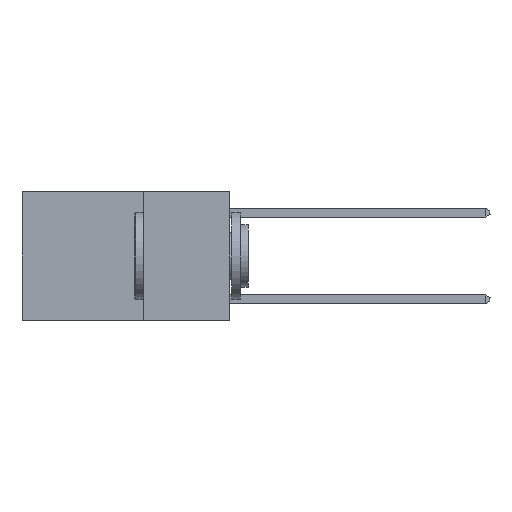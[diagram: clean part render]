
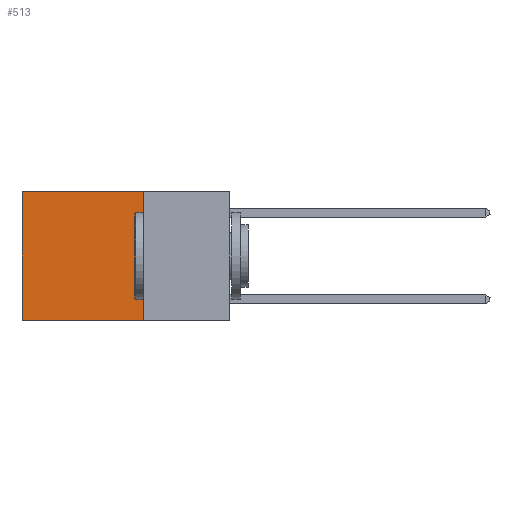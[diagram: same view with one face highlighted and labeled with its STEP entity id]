
A CAD part, left-side view. The second image highlights one B-rep face of the part: STEP entity #513.
In plain terms, the highlighted planar face has unit normal (-1, 0, 0).
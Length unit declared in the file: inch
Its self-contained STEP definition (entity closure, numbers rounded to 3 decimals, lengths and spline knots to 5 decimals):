
#238 = ORIENTED_EDGE ( 'NONE', *, *, #12191, .F. ) ;
#352 = AXIS2_PLACEMENT_3D ( 'NONE', #13266, #19711, #5676 ) ;
#513 = ADVANCED_FACE ( 'NONE', ( #18277 ), #3941, .F. ) ;
#777 = CARTESIAN_POINT ( 'NONE',  ( 0.2625, 0.25, 0. ) ) ;
#1265 = ORIENTED_EDGE ( 'NONE', *, *, #4638, .T. ) ;
#1633 = LINE ( 'NONE', #2740, #7583 ) ;
#2740 = CARTESIAN_POINT ( 'NONE',  ( 0.2625, 0.25, -0.37 ) ) ;
#3941 = PLANE ( 'NONE',  #352 ) ;
#4431 = CARTESIAN_POINT ( 'NONE',  ( 0.2625, 0.6, 0. ) ) ;
#4638 = EDGE_CURVE ( 'NONE', #11487, #13018, #13385, .T. ) ;
#4892 = VERTEX_POINT ( 'NONE', #7438 ) ;
#5676 = DIRECTION ( 'NONE',  ( 0., 0., -1. ) ) ;
#6156 = LINE ( 'NONE', #4431, #12904 ) ;
#6870 = LINE ( 'NONE', #19671, #14142 ) ;
#7267 = CARTESIAN_POINT ( 'NONE',  ( 0.2625, 0.25, 0. ) ) ;
#7438 = CARTESIAN_POINT ( 'NONE',  ( 0.2625, 0.25, -0.37 ) ) ;
#7583 = VECTOR ( 'NONE', #10833, 39.37008 ) ;
#8509 = DIRECTION ( 'NONE',  ( 0., 0., -1. ) ) ;
#9826 = ORIENTED_EDGE ( 'NONE', *, *, #12800, .F. ) ;
#10195 = DIRECTION ( 'NONE',  ( 0., 1., 0. ) ) ;
#10833 = DIRECTION ( 'NONE',  ( 0., 1., 0. ) ) ;
#11487 = VERTEX_POINT ( 'NONE', #7267 ) ;
#11897 = CARTESIAN_POINT ( 'NONE',  ( 0.2625, 0.6, -0.37 ) ) ;
#12191 = EDGE_CURVE ( 'NONE', #4892, #17804, #1633, .T. ) ;
#12800 = EDGE_CURVE ( 'NONE', #11487, #4892, #6870, .T. ) ;
#12904 = VECTOR ( 'NONE', #16892, 39.37008 ) ;
#13018 = VERTEX_POINT ( 'NONE', #18260 ) ;
#13266 = CARTESIAN_POINT ( 'NONE',  ( 0.2625, 0.25, 0. ) ) ;
#13385 = LINE ( 'NONE', #777, #17133 ) ;
#14142 = VECTOR ( 'NONE', #8509, 39.37008 ) ;
#14915 = ORIENTED_EDGE ( 'NONE', *, *, #14932, .T. ) ;
#14932 = EDGE_CURVE ( 'NONE', #13018, #17804, #6156, .T. ) ;
#15496 = EDGE_LOOP ( 'NONE', ( #14915, #238, #9826, #1265 ) ) ;
#16892 = DIRECTION ( 'NONE',  ( 0., 0., -1. ) ) ;
#17133 = VECTOR ( 'NONE', #10195, 39.37008 ) ;
#17804 = VERTEX_POINT ( 'NONE', #11897 ) ;
#18260 = CARTESIAN_POINT ( 'NONE',  ( 0.2625, 0.6, 0. ) ) ;
#18277 = FACE_OUTER_BOUND ( 'NONE', #15496, .T. ) ;
#19671 = CARTESIAN_POINT ( 'NONE',  ( 0.2625, 0.25, 0. ) ) ;
#19711 = DIRECTION ( 'NONE',  ( 1., 0., 0. ) ) ;
